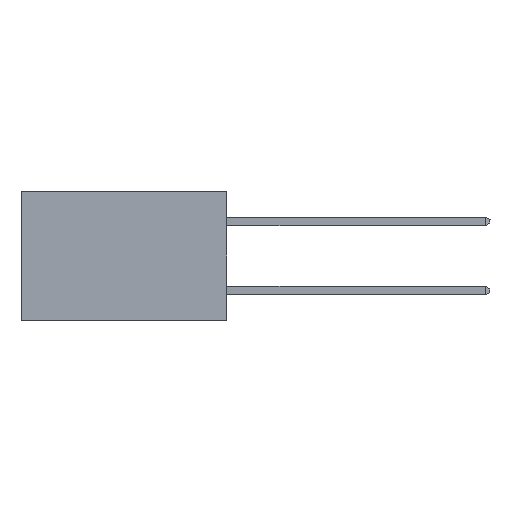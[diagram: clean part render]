
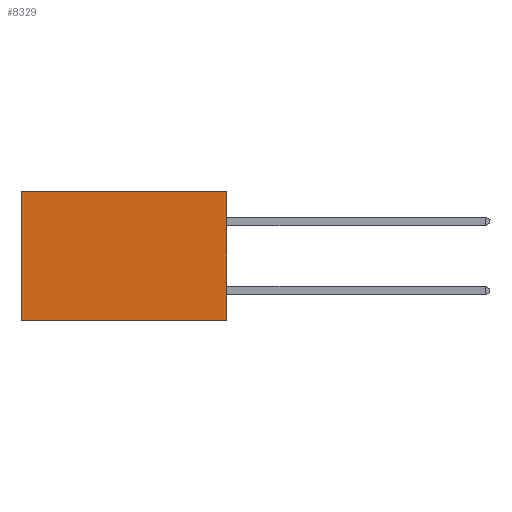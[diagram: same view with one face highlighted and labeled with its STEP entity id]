
A CAD part, left-side view. The second image highlights one B-rep face of the part: STEP entity #8329.
In plain terms, the highlighted planar face has unit normal (-1, 0, 0).
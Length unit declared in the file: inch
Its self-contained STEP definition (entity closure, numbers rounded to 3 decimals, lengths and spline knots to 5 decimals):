
#305 = VERTEX_POINT ( 'NONE', #7149 ) ;
#1152 = CARTESIAN_POINT ( 'NONE',  ( 0.277, 0., -0.37 ) ) ;
#1310 = ORIENTED_EDGE ( 'NONE', *, *, #10523, .T. ) ;
#1656 = ORIENTED_EDGE ( 'NONE', *, *, #12155, .F. ) ;
#2322 = DIRECTION ( 'NONE',  ( 1., 0., 0. ) ) ;
#2634 = LINE ( 'NONE', #2843, #5321 ) ;
#2775 = VECTOR ( 'NONE', #12528, 39.37008 ) ;
#2843 = CARTESIAN_POINT ( 'NONE',  ( 0.277, 0.59, -0.37 ) ) ;
#3244 = CARTESIAN_POINT ( 'NONE',  ( 0.277, 0., -0.37 ) ) ;
#4348 = ORIENTED_EDGE ( 'NONE', *, *, #14403, .F. ) ;
#4715 = ORIENTED_EDGE ( 'NONE', *, *, #13272, .T. ) ;
#5134 = CARTESIAN_POINT ( 'NONE',  ( 0.277, 0., 0. ) ) ;
#5321 = VECTOR ( 'NONE', #14119, 39.37008 ) ;
#6292 = VECTOR ( 'NONE', #12005, 39.37008 ) ;
#6459 = AXIS2_PLACEMENT_3D ( 'NONE', #9154, #2322, #10305 ) ;
#6682 = VERTEX_POINT ( 'NONE', #3244 ) ;
#7149 = CARTESIAN_POINT ( 'NONE',  ( 0.277, 0.59, -0.37 ) ) ;
#7368 = VERTEX_POINT ( 'NONE', #13427 ) ;
#8329 = ADVANCED_FACE ( 'NONE', ( #13495 ), #9196, .F. ) ;
#8871 = LINE ( 'NONE', #1152, #2775 ) ;
#9143 = EDGE_LOOP ( 'NONE', ( #1310, #4348, #1656, #4715 ) ) ;
#9154 = CARTESIAN_POINT ( 'NONE',  ( 0.277, 0., -0.37 ) ) ;
#9196 = PLANE ( 'NONE',  #6459 ) ;
#10031 = DIRECTION ( 'NONE',  ( 0., 1., 0. ) ) ;
#10305 = DIRECTION ( 'NONE',  ( 0., 0., -1. ) ) ;
#10523 = EDGE_CURVE ( 'NONE', #7368, #305, #2634, .T. ) ;
#10876 = CARTESIAN_POINT ( 'NONE',  ( 0.277, 0., 0. ) ) ;
#11236 = VECTOR ( 'NONE', #10031, 39.37008 ) ;
#12005 = DIRECTION ( 'NONE',  ( 0., 1., 0. ) ) ;
#12155 = EDGE_CURVE ( 'NONE', #12571, #6682, #8871, .T. ) ;
#12336 = LINE ( 'NONE', #10876, #6292 ) ;
#12528 = DIRECTION ( 'NONE',  ( 0., 0., -1. ) ) ;
#12571 = VERTEX_POINT ( 'NONE', #5134 ) ;
#13272 = EDGE_CURVE ( 'NONE', #12571, #7368, #12336, .T. ) ;
#13354 = CARTESIAN_POINT ( 'NONE',  ( 0.277, 0., -0.37 ) ) ;
#13427 = CARTESIAN_POINT ( 'NONE',  ( 0.277, 0.59, 0. ) ) ;
#13495 = FACE_OUTER_BOUND ( 'NONE', #9143, .T. ) ;
#14119 = DIRECTION ( 'NONE',  ( 0., 0., -1. ) ) ;
#14225 = LINE ( 'NONE', #13354, #11236 ) ;
#14403 = EDGE_CURVE ( 'NONE', #6682, #305, #14225, .T. ) ;
